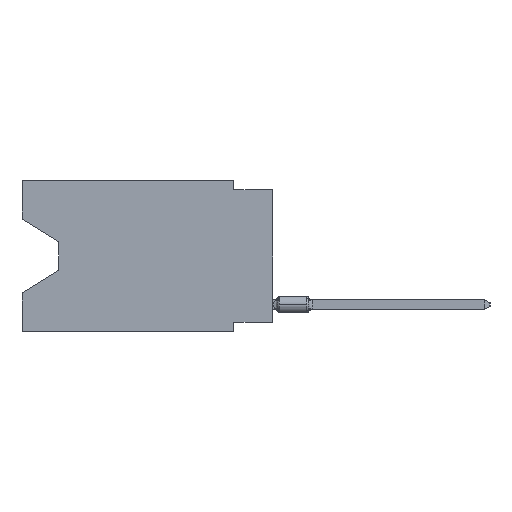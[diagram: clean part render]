
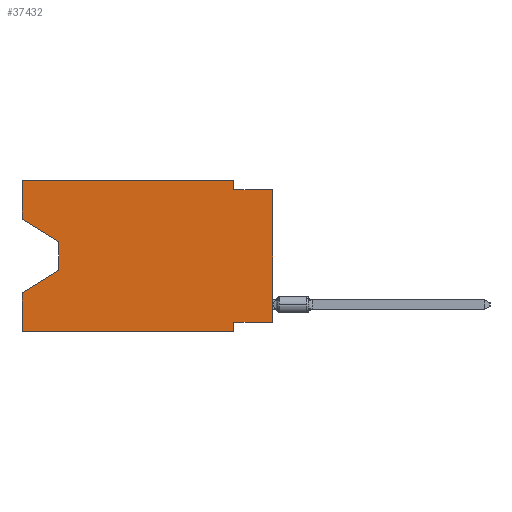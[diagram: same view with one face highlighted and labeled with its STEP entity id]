
A CAD part, left-side view. The second image highlights one B-rep face of the part: STEP entity #37432.
In plain terms, the highlighted planar face has unit normal (-1, 0, 0).
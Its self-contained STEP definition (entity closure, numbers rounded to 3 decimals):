
#547 = DIRECTION ( 'NONE',  ( 0., 0., -1. ) ) ;
#632 = VERTEX_POINT ( 'NONE', #8852 ) ;
#1075 = LINE ( 'NONE', #1601, #14728 ) ;
#1340 = VECTOR ( 'NONE', #42072, 1000. ) ;
#1601 = CARTESIAN_POINT ( 'NONE',  ( 0., 0., -9.271 ) ) ;
#2543 = VERTEX_POINT ( 'NONE', #22145 ) ;
#2549 = DIRECTION ( 'NONE',  ( 0., 0., 1. ) ) ;
#3131 = DIRECTION ( 'NONE',  ( 0., 0., -1. ) ) ;
#3672 = CARTESIAN_POINT ( 'NONE',  ( 0., 13.97, -5.893 ) ) ;
#3756 = VECTOR ( 'NONE', #2549, 1000. ) ;
#3766 = CARTESIAN_POINT ( 'NONE',  ( 0., 13.97, -4.013 ) ) ;
#5181 = VECTOR ( 'NONE', #29503, 1000. ) ;
#5431 = PLANE ( 'NONE',  #12776 ) ;
#5479 = VERTEX_POINT ( 'NONE', #44110 ) ;
#5965 = VECTOR ( 'NONE', #3131, 1000. ) ;
#7767 = VERTEX_POINT ( 'NONE', #17022 ) ;
#8639 = CARTESIAN_POINT ( 'NONE',  ( 0., 2.54, 0. ) ) ;
#8852 = CARTESIAN_POINT ( 'NONE',  ( 0., 16.383, -9.906 ) ) ;
#8903 = EDGE_CURVE ( 'NONE', #7767, #32097, #19704, .T. ) ;
#8998 = CARTESIAN_POINT ( 'NONE',  ( 0., 2.54, -9.271 ) ) ;
#9633 = LINE ( 'NONE', #25871, #1340 ) ;
#10080 = LINE ( 'NONE', #39069, #5965 ) ;
#10115 = CARTESIAN_POINT ( 'NONE',  ( 0., 16.383, -2.546 ) ) ;
#10128 = EDGE_LOOP ( 'NONE', ( #46642, #33865, #38072, #41297, #38013, #31860, #40473, #29433, #32448, #17831, #49001, #35221 ) ) ;
#11053 = LINE ( 'NONE', #21539, #3756 ) ;
#11190 = VECTOR ( 'NONE', #29415, 1000. ) ;
#11524 = EDGE_CURVE ( 'NONE', #17342, #32097, #11053, .T. ) ;
#11580 = DIRECTION ( 'NONE',  ( 0., 0., 1. ) ) ;
#12776 = AXIS2_PLACEMENT_3D ( 'NONE', #33874, #42117, #13647 ) ;
#13185 = LINE ( 'NONE', #33671, #11190 ) ;
#13273 = CARTESIAN_POINT ( 'NONE',  ( 0., 16.383, 0. ) ) ;
#13647 = DIRECTION ( 'NONE',  ( 0., 0., -1. ) ) ;
#13810 = CARTESIAN_POINT ( 'NONE',  ( 0., 13.97, -4.013 ) ) ;
#14103 = CARTESIAN_POINT ( 'NONE',  ( 0., 0., -0.635 ) ) ;
#14305 = VERTEX_POINT ( 'NONE', #8639 ) ;
#14728 = VECTOR ( 'NONE', #25029, 1000. ) ;
#14850 = EDGE_CURVE ( 'NONE', #35436, #5479, #10080, .T. ) ;
#15008 = VERTEX_POINT ( 'NONE', #3672 ) ;
#16478 = LINE ( 'NONE', #25443, #26364 ) ;
#16867 = DIRECTION ( 'NONE',  ( 0., -0.855, -0.519 ) ) ;
#16887 = FACE_OUTER_BOUND ( 'NONE', #10128, .T. ) ;
#17022 = CARTESIAN_POINT ( 'NONE',  ( 0., 2.54, -0.635 ) ) ;
#17216 = CARTESIAN_POINT ( 'NONE',  ( 0., 0., -9.271 ) ) ;
#17342 = VERTEX_POINT ( 'NONE', #17216 ) ;
#17831 = ORIENTED_EDGE ( 'NONE', *, *, #37033, .F. ) ;
#18723 = LINE ( 'NONE', #22450, #46821 ) ;
#19704 = LINE ( 'NONE', #19969, #36744 ) ;
#19969 = CARTESIAN_POINT ( 'NONE',  ( 0., 0., -0.635 ) ) ;
#21539 = CARTESIAN_POINT ( 'NONE',  ( 0., 0., 0. ) ) ;
#21812 = EDGE_CURVE ( 'NONE', #2543, #52313, #30332, .T. ) ;
#22079 = LINE ( 'NONE', #13810, #39395 ) ;
#22145 = CARTESIAN_POINT ( 'NONE',  ( 0., 16.383, -2.546 ) ) ;
#22450 = CARTESIAN_POINT ( 'NONE',  ( 0., 16.383, 0. ) ) ;
#22589 = EDGE_CURVE ( 'NONE', #15008, #41563, #13185, .T. ) ;
#23250 = CARTESIAN_POINT ( 'NONE',  ( 0., 16.383, 0. ) ) ;
#23339 = EDGE_CURVE ( 'NONE', #52313, #15008, #22079, .T. ) ;
#23830 = CARTESIAN_POINT ( 'NONE',  ( 0., 16.383, 0. ) ) ;
#24590 = EDGE_CURVE ( 'NONE', #17342, #35436, #1075, .T. ) ;
#25029 = DIRECTION ( 'NONE',  ( 0., 1., 0. ) ) ;
#25443 = CARTESIAN_POINT ( 'NONE',  ( 0., 2.54, 0. ) ) ;
#25485 = VECTOR ( 'NONE', #16867, 1000. ) ;
#25871 = CARTESIAN_POINT ( 'NONE',  ( 0., 16.383, -9.906 ) ) ;
#25978 = DIRECTION ( 'NONE',  ( 0., 0., -1. ) ) ;
#26364 = VECTOR ( 'NONE', #25978, 1000. ) ;
#29415 = DIRECTION ( 'NONE',  ( 0., 0.855, -0.519 ) ) ;
#29433 = ORIENTED_EDGE ( 'NONE', *, *, #11524, .T. ) ;
#29503 = DIRECTION ( 'NONE',  ( 0., 0., 1. ) ) ;
#30332 = LINE ( 'NONE', #10115, #25485 ) ;
#30831 = CARTESIAN_POINT ( 'NONE',  ( 0., 16.383, -7.36 ) ) ;
#31860 = ORIENTED_EDGE ( 'NONE', *, *, #14850, .F. ) ;
#32097 = VERTEX_POINT ( 'NONE', #14103 ) ;
#32448 = ORIENTED_EDGE ( 'NONE', *, *, #8903, .F. ) ;
#33671 = CARTESIAN_POINT ( 'NONE',  ( 0., 13.97, -5.893 ) ) ;
#33865 = ORIENTED_EDGE ( 'NONE', *, *, #23339, .T. ) ;
#33874 = CARTESIAN_POINT ( 'NONE',  ( 0., 16.383, 0. ) ) ;
#34368 = EDGE_CURVE ( 'NONE', #632, #41563, #48242, .T. ) ;
#35221 = ORIENTED_EDGE ( 'NONE', *, *, #44872, .F. ) ;
#35436 = VERTEX_POINT ( 'NONE', #8998 ) ;
#36192 = DIRECTION ( 'NONE',  ( 0., -1., 0. ) ) ;
#36744 = VECTOR ( 'NONE', #36192, 1000. ) ;
#37033 = EDGE_CURVE ( 'NONE', #14305, #7767, #16478, .T. ) ;
#37432 = ADVANCED_FACE ( 'NONE', ( #16887 ), #5431, .F. ) ;
#38013 = ORIENTED_EDGE ( 'NONE', *, *, #41090, .T. ) ;
#38072 = ORIENTED_EDGE ( 'NONE', *, *, #22589, .T. ) ;
#39069 = CARTESIAN_POINT ( 'NONE',  ( 0., 2.54, -9.906 ) ) ;
#39395 = VECTOR ( 'NONE', #547, 1000. ) ;
#40473 = ORIENTED_EDGE ( 'NONE', *, *, #24590, .F. ) ;
#40974 = VECTOR ( 'NONE', #11580, 1000. ) ;
#41090 = EDGE_CURVE ( 'NONE', #632, #5479, #9633, .T. ) ;
#41297 = ORIENTED_EDGE ( 'NONE', *, *, #34368, .F. ) ;
#41563 = VERTEX_POINT ( 'NONE', #30831 ) ;
#42072 = DIRECTION ( 'NONE',  ( 0., -1., 0. ) ) ;
#42117 = DIRECTION ( 'NONE',  ( 1., 0., 0. ) ) ;
#44110 = CARTESIAN_POINT ( 'NONE',  ( 0., 2.54, -9.906 ) ) ;
#44872 = EDGE_CURVE ( 'NONE', #2543, #48805, #49926, .T. ) ;
#45385 = EDGE_CURVE ( 'NONE', #48805, #14305, #18723, .T. ) ;
#46642 = ORIENTED_EDGE ( 'NONE', *, *, #21812, .T. ) ;
#46821 = VECTOR ( 'NONE', #51358, 1000. ) ;
#48242 = LINE ( 'NONE', #23830, #40974 ) ;
#48805 = VERTEX_POINT ( 'NONE', #23250 ) ;
#49001 = ORIENTED_EDGE ( 'NONE', *, *, #45385, .F. ) ;
#49926 = LINE ( 'NONE', #13273, #5181 ) ;
#51358 = DIRECTION ( 'NONE',  ( 0., -1., 0. ) ) ;
#52313 = VERTEX_POINT ( 'NONE', #3766 ) ;
